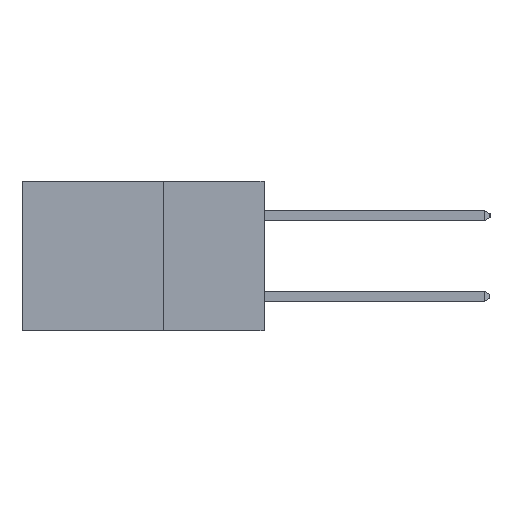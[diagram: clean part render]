
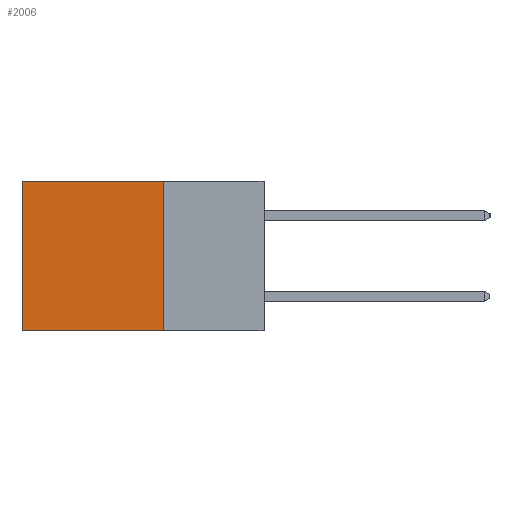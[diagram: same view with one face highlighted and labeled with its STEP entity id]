
A CAD part, left-side view. The second image highlights one B-rep face of the part: STEP entity #2006.
In plain terms, the highlighted planar face has unit normal (-1, 0, 0).
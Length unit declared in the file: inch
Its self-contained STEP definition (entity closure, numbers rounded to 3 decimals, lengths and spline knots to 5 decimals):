
#64 = DIRECTION ( 'NONE',  ( 0., 1., 0. ) ) ;
#540 = EDGE_CURVE ( 'NONE', #14743, #10239, #4111, .T. ) ;
#909 = VERTEX_POINT ( 'NONE', #6342 ) ;
#2006 = ADVANCED_FACE ( 'NONE', ( #4454 ), #4195, .F. ) ;
#2849 = VECTOR ( 'NONE', #4200, 39.37008 ) ;
#3154 = LINE ( 'NONE', #10063, #9401 ) ;
#3801 = AXIS2_PLACEMENT_3D ( 'NONE', #9947, #15477, #4286 ) ;
#4096 = EDGE_LOOP ( 'NONE', ( #17269, #10058, #12774, #12821 ) ) ;
#4111 = LINE ( 'NONE', #9859, #9118 ) ;
#4195 = PLANE ( 'NONE',  #3801 ) ;
#4200 = DIRECTION ( 'NONE',  ( 0., 0., -1. ) ) ;
#4286 = DIRECTION ( 'NONE',  ( 0., 0., -1. ) ) ;
#4454 = FACE_OUTER_BOUND ( 'NONE', #4096, .T. ) ;
#6342 = CARTESIAN_POINT ( 'NONE',  ( 0.2615, 0.6, 0. ) ) ;
#6873 = CARTESIAN_POINT ( 'NONE',  ( 0.2615, 0.25, 0. ) ) ;
#6969 = CARTESIAN_POINT ( 'NONE',  ( 0.2615, 0.25, 0. ) ) ;
#9022 = VERTEX_POINT ( 'NONE', #11044 ) ;
#9118 = VECTOR ( 'NONE', #16743, 39.37008 ) ;
#9343 = LINE ( 'NONE', #14878, #2849 ) ;
#9401 = VECTOR ( 'NONE', #16943, 39.37008 ) ;
#9590 = LINE ( 'NONE', #6969, #9982 ) ;
#9859 = CARTESIAN_POINT ( 'NONE',  ( 0.2615, 0.25, -0.37 ) ) ;
#9947 = CARTESIAN_POINT ( 'NONE',  ( 0.2615, 0.25, -0.37 ) ) ;
#9982 = VECTOR ( 'NONE', #64, 39.37008 ) ;
#10058 = ORIENTED_EDGE ( 'NONE', *, *, #17079, .F. ) ;
#10063 = CARTESIAN_POINT ( 'NONE',  ( 0.2615, 0.25, -0.37 ) ) ;
#10239 = VERTEX_POINT ( 'NONE', #11970 ) ;
#11044 = CARTESIAN_POINT ( 'NONE',  ( 0.2615, 0.6, -0.37 ) ) ;
#11970 = CARTESIAN_POINT ( 'NONE',  ( 0.2615, 0.25, -0.37 ) ) ;
#12774 = ORIENTED_EDGE ( 'NONE', *, *, #540, .F. ) ;
#12821 = ORIENTED_EDGE ( 'NONE', *, *, #16157, .T. ) ;
#14293 = EDGE_CURVE ( 'NONE', #909, #9022, #9343, .T. ) ;
#14743 = VERTEX_POINT ( 'NONE', #6873 ) ;
#14878 = CARTESIAN_POINT ( 'NONE',  ( 0.2615, 0.6, -0.37 ) ) ;
#15477 = DIRECTION ( 'NONE',  ( 1., 0., 0. ) ) ;
#16157 = EDGE_CURVE ( 'NONE', #14743, #909, #9590, .T. ) ;
#16743 = DIRECTION ( 'NONE',  ( 0., 0., -1. ) ) ;
#16943 = DIRECTION ( 'NONE',  ( 0., 1., 0. ) ) ;
#17079 = EDGE_CURVE ( 'NONE', #10239, #9022, #3154, .T. ) ;
#17269 = ORIENTED_EDGE ( 'NONE', *, *, #14293, .T. ) ;
